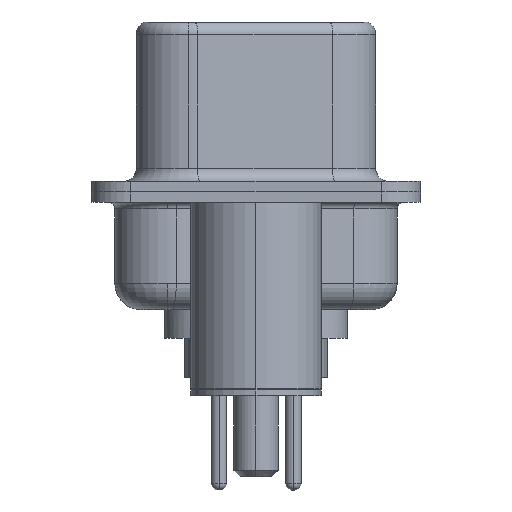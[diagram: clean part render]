
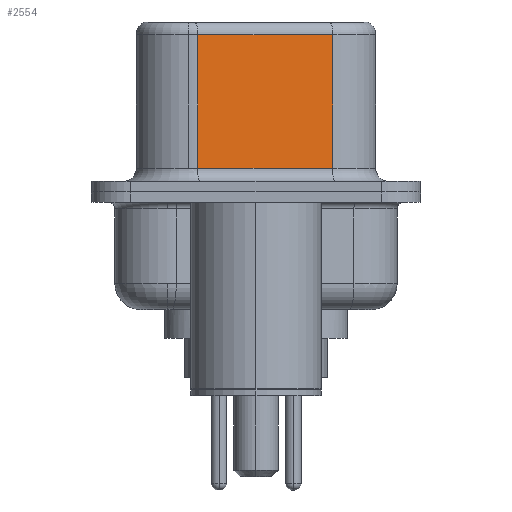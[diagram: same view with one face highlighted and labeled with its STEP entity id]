
A CAD part, left-side view. The second image highlights one B-rep face of the part: STEP entity #2554.
In plain terms, the highlighted planar face has unit normal (-0.985, -0.174, 0).
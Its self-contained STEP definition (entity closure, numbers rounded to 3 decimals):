
#391 = CARTESIAN_POINT ( 'NONE',  ( 3.675, 2.233, 0.9 ) ) ;
#768 = EDGE_CURVE ( 'NONE', #12129, #18569, #14997, .T. ) ;
#1158 = DIRECTION ( 'NONE',  ( -0.174, 0.985, 0. ) ) ;
#2554 = ADVANCED_FACE ( 'NONE', ( #11366 ), #11332, .F. ) ;
#2894 = CARTESIAN_POINT ( 'NONE',  ( 3.675, 2.233, 6.02 ) ) ;
#3018 = VECTOR ( 'NONE', #15172, 1000. ) ;
#3266 = VECTOR ( 'NONE', #1158, 1000. ) ;
#3288 = ORIENTED_EDGE ( 'NONE', *, *, #6728, .T. ) ;
#3398 = VECTOR ( 'NONE', #16780, 1000. ) ;
#3480 = VECTOR ( 'NONE', #9256, 1000. ) ;
#3855 = LINE ( 'NONE', #10959, #3398 ) ;
#6128 = CARTESIAN_POINT ( 'NONE',  ( 4.585, -2.927, 6.02 ) ) ;
#6341 = CARTESIAN_POINT ( 'NONE',  ( 4.585, -2.927, 0.9 ) ) ;
#6389 = AXIS2_PLACEMENT_3D ( 'NONE', #8509, #11531, #11385 ) ;
#6725 = EDGE_CURVE ( 'NONE', #12129, #8291, #16053, .T. ) ;
#6728 = EDGE_CURVE ( 'NONE', #9337, #8291, #10783, .T. ) ;
#8291 = VERTEX_POINT ( 'NONE', #12896 ) ;
#8509 = CARTESIAN_POINT ( 'NONE',  ( 4.585, -2.927, 6.52 ) ) ;
#9256 = DIRECTION ( 'NONE',  ( 0., 0., -1. ) ) ;
#9337 = VERTEX_POINT ( 'NONE', #391 ) ;
#10783 = LINE ( 'NONE', #6341, #3018 ) ;
#10959 = CARTESIAN_POINT ( 'NONE',  ( 3.675, 2.233, 6.52 ) ) ;
#11332 = PLANE ( 'NONE',  #6389 ) ;
#11366 = FACE_OUTER_BOUND ( 'NONE', #13557, .T. ) ;
#11385 = DIRECTION ( 'NONE',  ( -0.174, 0.985, 0. ) ) ;
#11531 = DIRECTION ( 'NONE',  ( 0.985, 0.174, 0. ) ) ;
#12129 = VERTEX_POINT ( 'NONE', #17865 ) ;
#12713 = ORIENTED_EDGE ( 'NONE', *, *, #768, .T. ) ;
#12896 = CARTESIAN_POINT ( 'NONE',  ( 4.585, -2.927, 0.9 ) ) ;
#13557 = EDGE_LOOP ( 'NONE', ( #14342, #12713, #17381, #3288 ) ) ;
#14342 = ORIENTED_EDGE ( 'NONE', *, *, #6725, .F. ) ;
#14997 = LINE ( 'NONE', #6128, #3266 ) ;
#15172 = DIRECTION ( 'NONE',  ( 0.174, -0.985, 0. ) ) ;
#15451 = EDGE_CURVE ( 'NONE', #18569, #9337, #3855, .T. ) ;
#16053 = LINE ( 'NONE', #17945, #3480 ) ;
#16780 = DIRECTION ( 'NONE',  ( 0., 0., -1. ) ) ;
#17381 = ORIENTED_EDGE ( 'NONE', *, *, #15451, .T. ) ;
#17865 = CARTESIAN_POINT ( 'NONE',  ( 4.585, -2.927, 6.02 ) ) ;
#17945 = CARTESIAN_POINT ( 'NONE',  ( 4.585, -2.927, 6.52 ) ) ;
#18569 = VERTEX_POINT ( 'NONE', #2894 ) ;
